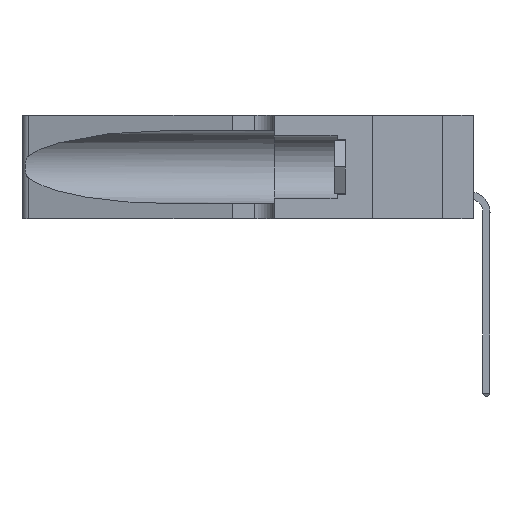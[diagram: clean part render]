
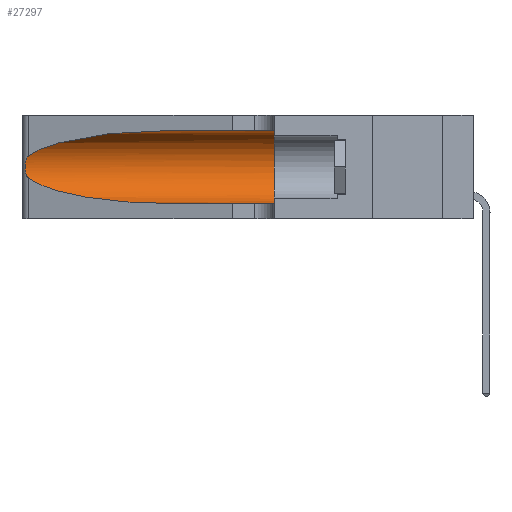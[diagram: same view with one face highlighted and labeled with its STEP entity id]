
A CAD part, left-side view. The second image highlights one B-rep face of the part: STEP entity #27297.
In plain terms, the highlighted cylindrical face has radius 3.308 mm (diameter 6.617 mm), a partial arc.
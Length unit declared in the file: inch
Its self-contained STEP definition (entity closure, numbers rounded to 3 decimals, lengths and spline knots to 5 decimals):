
#749 = FACE_OUTER_BOUND ( 'NONE', #18107, .T. ) ;
#2106 = CARTESIAN_POINT ( 'NONE',  ( 0.25487, 1.22718, 0.22369 ) ) ;
#2548 = CARTESIAN_POINT ( 'NONE',  ( 0.18966, 0.96281, 0.31525 ) ) ;
#3003 = DIRECTION ( 'NONE',  ( 0., -1., 0. ) ) ;
#3140 = CARTESIAN_POINT ( 'NONE',  ( 0.1305, 1.61858, 0.31525 ) ) ;
#3581 = EDGE_CURVE ( 'NONE', #7253, #11035, #9448, .T. ) ;
#4595 = DIRECTION ( 'NONE',  ( 0., 1., 0. ) ) ;
#4929 = CARTESIAN_POINT ( 'NONE',  ( 0.25639, 1.23184, 0.21858 ) ) ;
#5488 = CARTESIAN_POINT ( 'NONE',  ( 0.2373, 1.15595, 0.28018 ) ) ;
#5773 = AXIS2_PLACEMENT_3D ( 'NONE', #11867, #3003, #33850 ) ;
#7253 = VERTEX_POINT ( 'NONE', #30816 ) ;
#8687 = CARTESIAN_POINT ( 'NONE',  ( 0.1305, 0.72297, 0.05475 ) ) ;
#8934 = DIRECTION ( 'NONE',  ( 0., -1., 0. ) ) ;
#9448 = LINE ( 'NONE', #3140, #19560 ) ;
#10764 = CARTESIAN_POINT ( 'NONE',  ( 0.1305, 0.35, 0.185 ) ) ;
#11035 = VERTEX_POINT ( 'NONE', #19364 ) ;
#11333 = EDGE_CURVE ( 'NONE', #29877, #29027, #26145, .T. ) ;
#11867 = CARTESIAN_POINT ( 'NONE',  ( 0.1305, 1.61858, 0.185 ) ) ;
#13053 = CARTESIAN_POINT ( 'NONE',  ( 0.25787, 1.23484, 0.2124 ) ) ;
#13316 = CARTESIAN_POINT ( 'NONE',  ( 0.25555, 1.22994, 0.2215 ) ) ;
#13407 = CARTESIAN_POINT ( 'NONE',  ( 0.25487, 1.22718, 0.22369 ) ) ;
#14237 = DIRECTION ( 'NONE',  ( 0., -1., 0. ) ) ;
#15276 = CARTESIAN_POINT ( 'NONE',  ( 0.25487, 1.22718, 0.14631 ) ) ;
#15886 = CARTESIAN_POINT ( 'NONE',  ( 0.25854, 1.2359, 0.20912 ) ) ;
#16001 = CARTESIAN_POINT ( 'NONE',  ( 0.26017, 1.23833, 0.17102 ) ) ;
#16127 = CARTESIAN_POINT ( 'NONE',  ( 0.25555, 1.22993, 0.14849 ) ) ;
#16239 = EDGE_CURVE ( 'NONE', #7253, #22654, #27283, .T. ) ;
#17062 = CYLINDRICAL_SURFACE ( 'NONE', #5773, 0.13025 ) ;
#18107 = EDGE_LOOP ( 'NONE', ( #30500, #24702, #29164, #29251, #35726, #24343 ) ) ;
#19155 = CARTESIAN_POINT ( 'NONE',  ( 0.1305, 0.72297, 0.31525 ) ) ;
#19364 = CARTESIAN_POINT ( 'NONE',  ( 0.1305, 0.35, 0.31525 ) ) ;
#19560 = VECTOR ( 'NONE', #8934, 39.37008 ) ;
#20400 = AXIS2_PLACEMENT_3D ( 'NONE', #10764, #4595, #27197 ) ;
#20767 = B_SPLINE_CURVE_WITH_KNOTS ( 'NONE', 3,
 ( #2106, #13316, #4929, #13053, #15886, #32952, #26916, #21655, #16001, #29858, #32708, #24101, #16127, #35328 ),
 .UNSPECIFIED., .F., .F.,
 ( 4, 2, 2, 2, 2, 2, 4 ),
 ( 0., 0.00027, 0.00053, 0.00107, 0.0016, 0.00187, 0.00214 ),
 .UNSPECIFIED. ) ;
#21253 = EDGE_CURVE ( 'NONE', #22654, #29877, #20767, .T. ) ;
#21425 = CARTESIAN_POINT ( 'NONE',  ( 0.25487, 1.22718, 0.14631 ) ) ;
#21655 = CARTESIAN_POINT ( 'NONE',  ( 0.26075, 1.23896, 0.178 ) ) ;
#22654 = VERTEX_POINT ( 'NONE', #30026 ) ;
#23880 = EDGE_CURVE ( 'NONE', #29027, #23932, #31834, .T. ) ;
#23932 = VERTEX_POINT ( 'NONE', #32893 ) ;
#24101 = CARTESIAN_POINT ( 'NONE',  ( 0.25639, 1.23186, 0.15144 ) ) ;
#24343 = ORIENTED_EDGE ( 'NONE', *, *, #3581, .F. ) ;
#24485 = CARTESIAN_POINT ( 'NONE',  ( 0.2373, 1.15595, 0.08982 ) ) ;
#24702 = ORIENTED_EDGE ( 'NONE', *, *, #21253, .T. ) ;
#25215 = VECTOR ( 'NONE', #14237, 39.37008 ) ;
#26145 =( BOUNDED_CURVE ( )  B_SPLINE_CURVE ( 3, ( #21425, #24485, #35460, #32599 ),
 .UNSPECIFIED., .F., .F. ) 
 B_SPLINE_CURVE_WITH_KNOTS ( ( 4, 4 ),
 ( 3.44316, 4.71239 ),
 .UNSPECIFIED. ) 
 CURVE ( )  GEOMETRIC_REPRESENTATION_ITEM ( )  RATIONAL_B_SPLINE_CURVE ( ( 1., 0.87, 0.87, 1. ) ) 
 REPRESENTATION_ITEM ( '' )  );
#26916 = CARTESIAN_POINT ( 'NONE',  ( 0.26075, 1.23896, 0.19203 ) ) ;
#27197 = DIRECTION ( 'NONE',  ( 0., 0., 1. ) ) ;
#27283 =( BOUNDED_CURVE ( )  B_SPLINE_CURVE ( 3, ( #19155, #2548, #5488, #13407 ),
 .UNSPECIFIED., .F., .F. ) 
 B_SPLINE_CURVE_WITH_KNOTS ( ( 4, 4 ),
 ( 1.5708, 2.84003 ),
 .UNSPECIFIED. ) 
 CURVE ( )  GEOMETRIC_REPRESENTATION_ITEM ( )  RATIONAL_B_SPLINE_CURVE ( ( 1., 0.87, 0.87, 1. ) ) 
 REPRESENTATION_ITEM ( '' )  );
#27297 = ADVANCED_FACE ( 'NONE', ( #749 ), #17062, .F. ) ;
#29027 = VERTEX_POINT ( 'NONE', #8687 ) ;
#29164 = ORIENTED_EDGE ( 'NONE', *, *, #11333, .T. ) ;
#29251 = ORIENTED_EDGE ( 'NONE', *, *, #23880, .T. ) ;
#29304 = EDGE_CURVE ( 'NONE', #11035, #23932, #30898, .T. ) ;
#29858 = CARTESIAN_POINT ( 'NONE',  ( 0.25856, 1.23593, 0.16098 ) ) ;
#29877 = VERTEX_POINT ( 'NONE', #15276 ) ;
#30026 = CARTESIAN_POINT ( 'NONE',  ( 0.25487, 1.22718, 0.22369 ) ) ;
#30065 = CARTESIAN_POINT ( 'NONE',  ( 0.1305, 1.61858, 0.05475 ) ) ;
#30500 = ORIENTED_EDGE ( 'NONE', *, *, #16239, .T. ) ;
#30816 = CARTESIAN_POINT ( 'NONE',  ( 0.1305, 0.72297, 0.31525 ) ) ;
#30898 = CIRCLE ( 'NONE', #20400, 0.13025 ) ;
#31834 = LINE ( 'NONE', #30065, #25215 ) ;
#32599 = CARTESIAN_POINT ( 'NONE',  ( 0.1305, 0.72297, 0.05475 ) ) ;
#32708 = CARTESIAN_POINT ( 'NONE',  ( 0.25789, 1.23486, 0.15765 ) ) ;
#32893 = CARTESIAN_POINT ( 'NONE',  ( 0.1305, 0.35, 0.05475 ) ) ;
#32952 = CARTESIAN_POINT ( 'NONE',  ( 0.26018, 1.23835, 0.19895 ) ) ;
#33850 = DIRECTION ( 'NONE',  ( 0., 0., -1. ) ) ;
#35328 = CARTESIAN_POINT ( 'NONE',  ( 0.25487, 1.22718, 0.14631 ) ) ;
#35460 = CARTESIAN_POINT ( 'NONE',  ( 0.18966, 0.96281, 0.05475 ) ) ;
#35726 = ORIENTED_EDGE ( 'NONE', *, *, #29304, .F. ) ;
